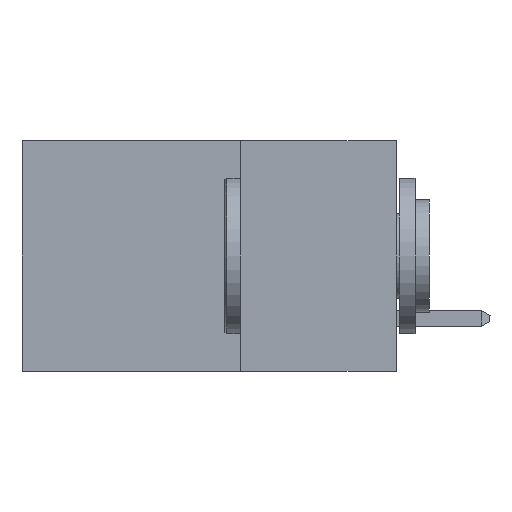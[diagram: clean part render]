
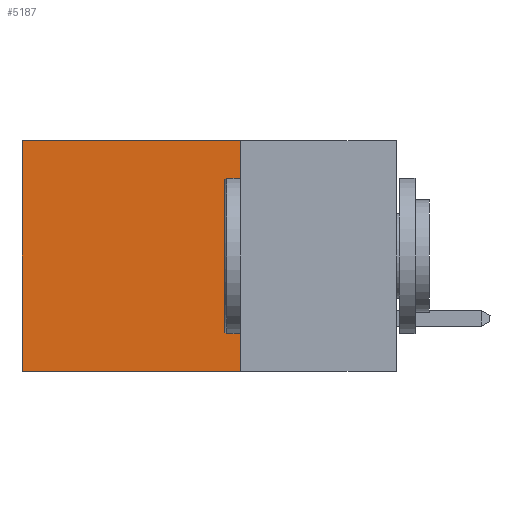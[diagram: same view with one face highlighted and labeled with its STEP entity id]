
A CAD part, left-side view. The second image highlights one B-rep face of the part: STEP entity #5187.
In plain terms, the highlighted planar face has unit normal (-1, 0, 0).
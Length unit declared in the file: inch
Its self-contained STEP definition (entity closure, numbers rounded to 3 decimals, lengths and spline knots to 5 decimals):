
#408 = FACE_OUTER_BOUND ( 'NONE', #17370, .T. ) ;
#1217 = DIRECTION ( 'NONE',  ( 0., 1., 0. ) ) ;
#1772 = CARTESIAN_POINT ( 'NONE',  ( 0.298, 0.25, -0.37 ) ) ;
#1873 = LINE ( 'NONE', #3288, #21894 ) ;
#2785 = EDGE_CURVE ( 'NONE', #22892, #12654, #1873, .T. ) ;
#2808 = VERTEX_POINT ( 'NONE', #17358 ) ;
#3288 = CARTESIAN_POINT ( 'NONE',  ( 0.298, 0.25, 0. ) ) ;
#4106 = EDGE_CURVE ( 'NONE', #2808, #25066, #20018, .T. ) ;
#4788 = DIRECTION ( 'NONE',  ( 0., 0., -1. ) ) ;
#5187 = ADVANCED_FACE ( 'NONE', ( #408 ), #6453, .F. ) ;
#5342 = DIRECTION ( 'NONE',  ( 0., 1., 0. ) ) ;
#5755 = DIRECTION ( 'NONE',  ( 0., 0., -1. ) ) ;
#6328 = LINE ( 'NONE', #23243, #23023 ) ;
#6453 = PLANE ( 'NONE',  #23432 ) ;
#8464 = ORIENTED_EDGE ( 'NONE', *, *, #4106, .F. ) ;
#12337 = CARTESIAN_POINT ( 'NONE',  ( 0.298, 0.25, 0. ) ) ;
#12379 = CARTESIAN_POINT ( 'NONE',  ( 0.298, 0.6, -0.37 ) ) ;
#12654 = VERTEX_POINT ( 'NONE', #24144 ) ;
#12767 = VECTOR ( 'NONE', #5342, 39.37008 ) ;
#14552 = CARTESIAN_POINT ( 'NONE',  ( 0.298, 0.25, 0. ) ) ;
#14963 = EDGE_CURVE ( 'NONE', #12654, #25066, #6328, .T. ) ;
#15495 = ORIENTED_EDGE ( 'NONE', *, *, #2785, .T. ) ;
#16597 = DIRECTION ( 'NONE',  ( 0., 0., -1. ) ) ;
#16611 = LINE ( 'NONE', #17946, #17220 ) ;
#16987 = ORIENTED_EDGE ( 'NONE', *, *, #14963, .T. ) ;
#17220 = VECTOR ( 'NONE', #16597, 39.37008 ) ;
#17358 = CARTESIAN_POINT ( 'NONE',  ( 0.298, 0.25, -0.37 ) ) ;
#17370 = EDGE_LOOP ( 'NONE', ( #16987, #8464, #20860, #15495 ) ) ;
#17946 = CARTESIAN_POINT ( 'NONE',  ( 0.298, 0.25, 0. ) ) ;
#18279 = DIRECTION ( 'NONE',  ( 1., 0., 0. ) ) ;
#20018 = LINE ( 'NONE', #1772, #12767 ) ;
#20860 = ORIENTED_EDGE ( 'NONE', *, *, #22599, .F. ) ;
#21894 = VECTOR ( 'NONE', #1217, 39.37008 ) ;
#22599 = EDGE_CURVE ( 'NONE', #22892, #2808, #16611, .T. ) ;
#22892 = VERTEX_POINT ( 'NONE', #14552 ) ;
#23023 = VECTOR ( 'NONE', #5755, 39.37008 ) ;
#23243 = CARTESIAN_POINT ( 'NONE',  ( 0.298, 0.6, 0. ) ) ;
#23432 = AXIS2_PLACEMENT_3D ( 'NONE', #12337, #18279, #4788 ) ;
#24144 = CARTESIAN_POINT ( 'NONE',  ( 0.298, 0.6, 0. ) ) ;
#25066 = VERTEX_POINT ( 'NONE', #12379 ) ;
